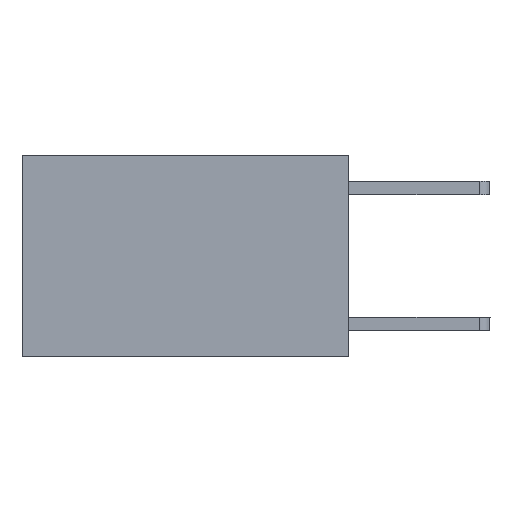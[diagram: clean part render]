
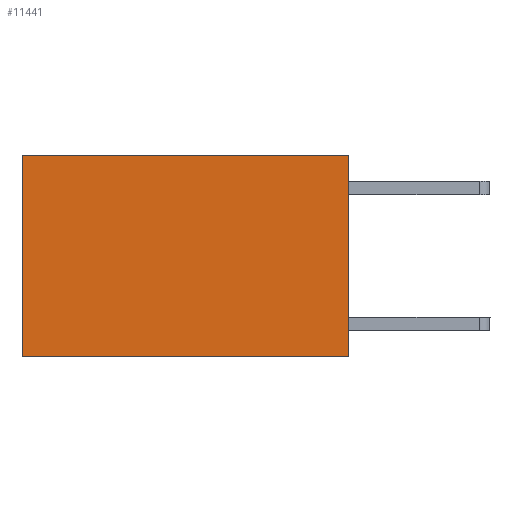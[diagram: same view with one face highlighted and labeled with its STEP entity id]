
A CAD part, left-side view. The second image highlights one B-rep face of the part: STEP entity #11441.
In plain terms, the highlighted planar face has unit normal (-1, 0, 0).
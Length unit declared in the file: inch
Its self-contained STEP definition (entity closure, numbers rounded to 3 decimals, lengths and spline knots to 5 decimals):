
#489 = VECTOR ( 'NONE', #1393, 39.37008 ) ;
#872 = AXIS2_PLACEMENT_3D ( 'NONE', #7369, #9329, #3305 ) ;
#1296 = CARTESIAN_POINT ( 'NONE',  ( 0.2625, 0.6, -0.37 ) ) ;
#1393 = DIRECTION ( 'NONE',  ( 0., 0., -1. ) ) ;
#1621 = EDGE_CURVE ( 'NONE', #3297, #4218, #9772, .T. ) ;
#2020 = VERTEX_POINT ( 'NONE', #9549 ) ;
#2173 = LINE ( 'NONE', #8862, #10066 ) ;
#2630 = ORIENTED_EDGE ( 'NONE', *, *, #8543, .F. ) ;
#2793 = DIRECTION ( 'NONE',  ( 0., 0., -1. ) ) ;
#2919 = DIRECTION ( 'NONE',  ( 0., 1., 0. ) ) ;
#3068 = CARTESIAN_POINT ( 'NONE',  ( 0.2625, 0., -0.37 ) ) ;
#3297 = VERTEX_POINT ( 'NONE', #11653 ) ;
#3305 = DIRECTION ( 'NONE',  ( 0., 0., -1. ) ) ;
#3567 = ORIENTED_EDGE ( 'NONE', *, *, #10782, .T. ) ;
#4047 = ORIENTED_EDGE ( 'NONE', *, *, #1621, .F. ) ;
#4218 = VERTEX_POINT ( 'NONE', #1296 ) ;
#5632 = VECTOR ( 'NONE', #2919, 39.37008 ) ;
#5656 = FACE_OUTER_BOUND ( 'NONE', #10505, .T. ) ;
#5836 = LINE ( 'NONE', #9378, #489 ) ;
#6350 = EDGE_CURVE ( 'NONE', #9147, #2020, #8396, .T. ) ;
#7369 = CARTESIAN_POINT ( 'NONE',  ( 0.2625, 0., 0. ) ) ;
#8030 = CARTESIAN_POINT ( 'NONE',  ( 0.2625, 0., 0. ) ) ;
#8043 = ORIENTED_EDGE ( 'NONE', *, *, #6350, .T. ) ;
#8396 = LINE ( 'NONE', #8030, #5632 ) ;
#8543 = EDGE_CURVE ( 'NONE', #9147, #3297, #2173, .T. ) ;
#8862 = CARTESIAN_POINT ( 'NONE',  ( 0.2625, 0., 0. ) ) ;
#9147 = VERTEX_POINT ( 'NONE', #12126 ) ;
#9329 = DIRECTION ( 'NONE',  ( 1., 0., 0. ) ) ;
#9378 = CARTESIAN_POINT ( 'NONE',  ( 0.2625, 0.6, 0. ) ) ;
#9480 = VECTOR ( 'NONE', #11543, 39.37008 ) ;
#9549 = CARTESIAN_POINT ( 'NONE',  ( 0.2625, 0.6, 0. ) ) ;
#9772 = LINE ( 'NONE', #3068, #9480 ) ;
#10066 = VECTOR ( 'NONE', #2793, 39.37008 ) ;
#10505 = EDGE_LOOP ( 'NONE', ( #3567, #4047, #2630, #8043 ) ) ;
#10782 = EDGE_CURVE ( 'NONE', #2020, #4218, #5836, .T. ) ;
#11441 = ADVANCED_FACE ( 'NONE', ( #5656 ), #11935, .F. ) ;
#11543 = DIRECTION ( 'NONE',  ( 0., 1., 0. ) ) ;
#11653 = CARTESIAN_POINT ( 'NONE',  ( 0.2625, 0., -0.37 ) ) ;
#11935 = PLANE ( 'NONE',  #872 ) ;
#12126 = CARTESIAN_POINT ( 'NONE',  ( 0.2625, 0., 0. ) ) ;
